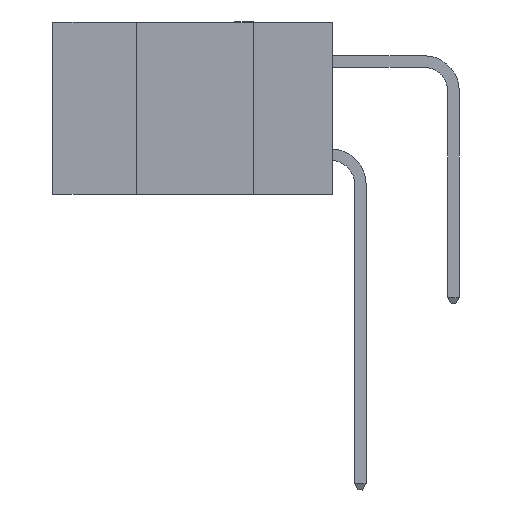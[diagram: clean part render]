
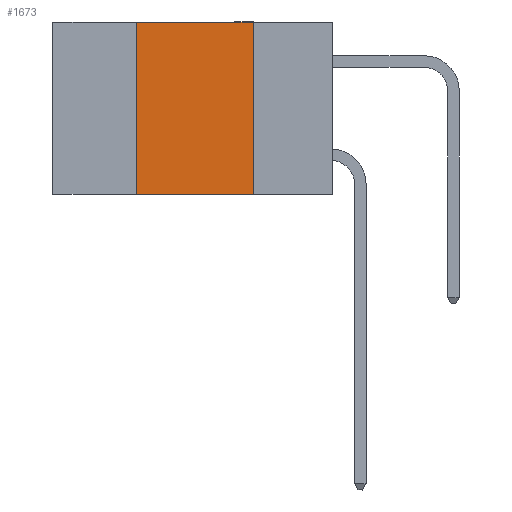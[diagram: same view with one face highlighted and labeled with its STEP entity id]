
A CAD part, left-side view. The second image highlights one B-rep face of the part: STEP entity #1673.
In plain terms, the highlighted planar face has unit normal (-1, 0, 0).
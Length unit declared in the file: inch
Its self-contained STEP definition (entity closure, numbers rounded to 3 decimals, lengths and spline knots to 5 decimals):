
#12 = CARTESIAN_POINT ( 'NONE',  ( 0., 0.17, -0.37 ) ) ;
#357 = LINE ( 'NONE', #6910, #10761 ) ;
#1013 = DIRECTION ( 'NONE',  ( 0., 0., -1. ) ) ;
#1121 = LINE ( 'NONE', #5515, #11532 ) ;
#1673 = ADVANCED_FACE ( 'NONE', ( #2440 ), #4221, .F. ) ;
#2110 = EDGE_CURVE ( 'NONE', #6126, #12903, #357, .T. ) ;
#2162 = DIRECTION ( 'NONE',  ( 0., 0., 1. ) ) ;
#2332 = LINE ( 'NONE', #13246, #5638 ) ;
#2440 = FACE_OUTER_BOUND ( 'NONE', #12714, .T. ) ;
#3584 = VECTOR ( 'NONE', #2162, 39.37008 ) ;
#3774 = CARTESIAN_POINT ( 'NONE',  ( 0., 0.42, 0. ) ) ;
#3948 = LINE ( 'NONE', #3774, #3584 ) ;
#4221 = PLANE ( 'NONE',  #6908 ) ;
#4341 = DIRECTION ( 'NONE',  ( 0., -1., 0. ) ) ;
#4689 = DIRECTION ( 'NONE',  ( 0., 0., -1. ) ) ;
#5515 = CARTESIAN_POINT ( 'NONE',  ( 0., 0.6, -0.37 ) ) ;
#5638 = VECTOR ( 'NONE', #4341, 39.37008 ) ;
#5886 = ORIENTED_EDGE ( 'NONE', *, *, #9065, .F. ) ;
#6126 = VERTEX_POINT ( 'NONE', #13275 ) ;
#6254 = ORIENTED_EDGE ( 'NONE', *, *, #9575, .T. ) ;
#6613 = DIRECTION ( 'NONE',  ( 0., -1., 0. ) ) ;
#6615 = CARTESIAN_POINT ( 'NONE',  ( 0., 0.6, 0. ) ) ;
#6908 = AXIS2_PLACEMENT_3D ( 'NONE', #6615, #12345, #1013 ) ;
#6910 = CARTESIAN_POINT ( 'NONE',  ( 0., 0.17, 0. ) ) ;
#6924 = CARTESIAN_POINT ( 'NONE',  ( 0., 0.42, 0. ) ) ;
#7910 = ORIENTED_EDGE ( 'NONE', *, *, #2110, .F. ) ;
#9065 = EDGE_CURVE ( 'NONE', #12548, #6126, #2332, .T. ) ;
#9369 = ORIENTED_EDGE ( 'NONE', *, *, #12030, .F. ) ;
#9575 = EDGE_CURVE ( 'NONE', #13149, #12903, #1121, .T. ) ;
#10761 = VECTOR ( 'NONE', #4689, 39.37008 ) ;
#11532 = VECTOR ( 'NONE', #6613, 39.37008 ) ;
#11927 = CARTESIAN_POINT ( 'NONE',  ( 0., 0.42, -0.37 ) ) ;
#12030 = EDGE_CURVE ( 'NONE', #13149, #12548, #3948, .T. ) ;
#12345 = DIRECTION ( 'NONE',  ( 1., 0., 0. ) ) ;
#12548 = VERTEX_POINT ( 'NONE', #6924 ) ;
#12714 = EDGE_LOOP ( 'NONE', ( #7910, #5886, #9369, #6254 ) ) ;
#12903 = VERTEX_POINT ( 'NONE', #12 ) ;
#13149 = VERTEX_POINT ( 'NONE', #11927 ) ;
#13246 = CARTESIAN_POINT ( 'NONE',  ( 0., 0.6, 0. ) ) ;
#13275 = CARTESIAN_POINT ( 'NONE',  ( 0., 0.17, 0. ) ) ;
